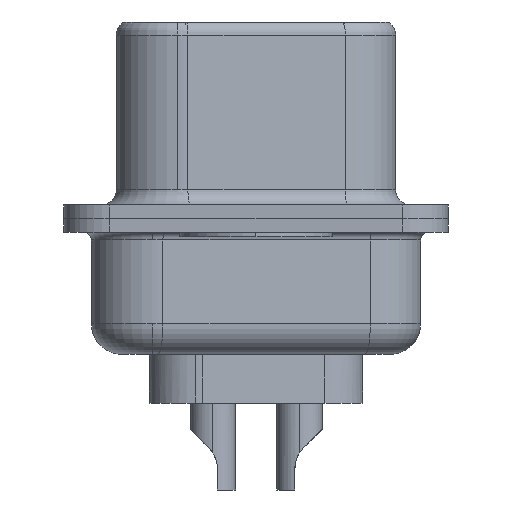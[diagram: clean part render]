
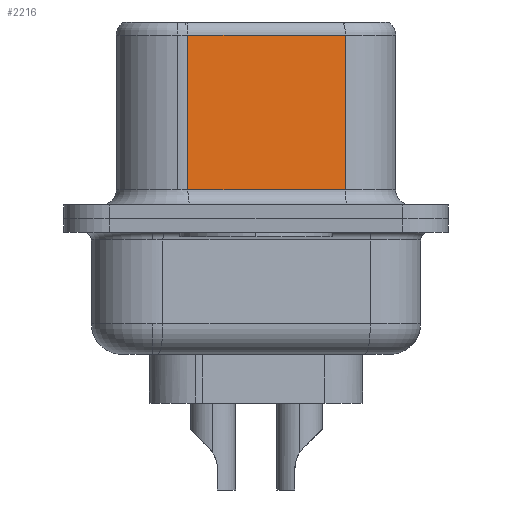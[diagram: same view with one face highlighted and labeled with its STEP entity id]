
A CAD part, left-side view. The second image highlights one B-rep face of the part: STEP entity #2216.
In plain terms, the highlighted planar face has unit normal (-0.985, -0.174, 0).
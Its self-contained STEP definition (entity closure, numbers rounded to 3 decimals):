
#1229 = CARTESIAN_POINT ( 'NONE',  ( 4.58, -2.927, 6.52 ) ) ;
#1764 = LINE ( 'NONE', #11712, #17972 ) ;
#2216 = ADVANCED_FACE ( 'NONE', ( #6184 ), #19849, .F. ) ;
#2362 = CARTESIAN_POINT ( 'NONE',  ( 4.58, -2.927, 6.52 ) ) ;
#2708 = ORIENTED_EDGE ( 'NONE', *, *, #14762, .T. ) ;
#3244 = DIRECTION ( 'NONE',  ( -0.174, 0.985, 0. ) ) ;
#3266 = DIRECTION ( 'NONE',  ( 0.174, -0.985, 0. ) ) ;
#3313 = VERTEX_POINT ( 'NONE', #16902 ) ;
#3805 = DIRECTION ( 'NONE',  ( 0., 0., -1. ) ) ;
#5174 = CARTESIAN_POINT ( 'NONE',  ( 4.58, -2.927, 0.95 ) ) ;
#6184 = FACE_OUTER_BOUND ( 'NONE', #6791, .T. ) ;
#6791 = EDGE_LOOP ( 'NONE', ( #22517, #13480, #2708, #13499 ) ) ;
#8220 = VERTEX_POINT ( 'NONE', #16971 ) ;
#8756 = VERTEX_POINT ( 'NONE', #10803 ) ;
#9245 = LINE ( 'NONE', #5174, #17116 ) ;
#10803 = CARTESIAN_POINT ( 'NONE',  ( 3.67, 2.233, 0.95 ) ) ;
#11356 = CARTESIAN_POINT ( 'NONE',  ( 4.58, -2.927, 6.02 ) ) ;
#11712 = CARTESIAN_POINT ( 'NONE',  ( 3.67, 2.233, 6.52 ) ) ;
#12195 = AXIS2_PLACEMENT_3D ( 'NONE', #2362, #17034, #3244 ) ;
#13480 = ORIENTED_EDGE ( 'NONE', *, *, #22762, .T. ) ;
#13499 = ORIENTED_EDGE ( 'NONE', *, *, #21653, .T. ) ;
#13905 = CARTESIAN_POINT ( 'NONE',  ( 4.58, -2.927, 0.95 ) ) ;
#14762 = EDGE_CURVE ( 'NONE', #3313, #8756, #1764, .T. ) ;
#15047 = EDGE_CURVE ( 'NONE', #8220, #16217, #22533, .T. ) ;
#15556 = VECTOR ( 'NONE', #19139, 1000. ) ;
#16217 = VERTEX_POINT ( 'NONE', #13905 ) ;
#16902 = CARTESIAN_POINT ( 'NONE',  ( 3.67, 2.233, 6.02 ) ) ;
#16971 = CARTESIAN_POINT ( 'NONE',  ( 4.58, -2.927, 6.02 ) ) ;
#17034 = DIRECTION ( 'NONE',  ( 0.985, 0.174, 0. ) ) ;
#17116 = VECTOR ( 'NONE', #3266, 1000. ) ;
#17972 = VECTOR ( 'NONE', #3805, 1000. ) ;
#19139 = DIRECTION ( 'NONE',  ( -0.174, 0.985, 0. ) ) ;
#19849 = PLANE ( 'NONE',  #12195 ) ;
#20008 = VECTOR ( 'NONE', #20625, 1000. ) ;
#20625 = DIRECTION ( 'NONE',  ( 0., 0., -1. ) ) ;
#21054 = LINE ( 'NONE', #11356, #15556 ) ;
#21653 = EDGE_CURVE ( 'NONE', #8756, #16217, #9245, .T. ) ;
#22517 = ORIENTED_EDGE ( 'NONE', *, *, #15047, .F. ) ;
#22533 = LINE ( 'NONE', #1229, #20008 ) ;
#22762 = EDGE_CURVE ( 'NONE', #8220, #3313, #21054, .T. ) ;
